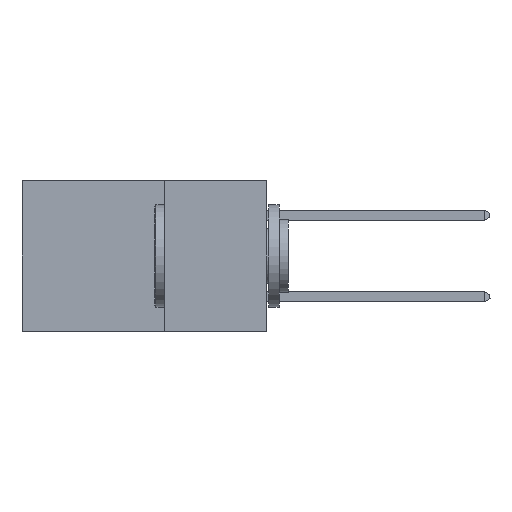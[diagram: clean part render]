
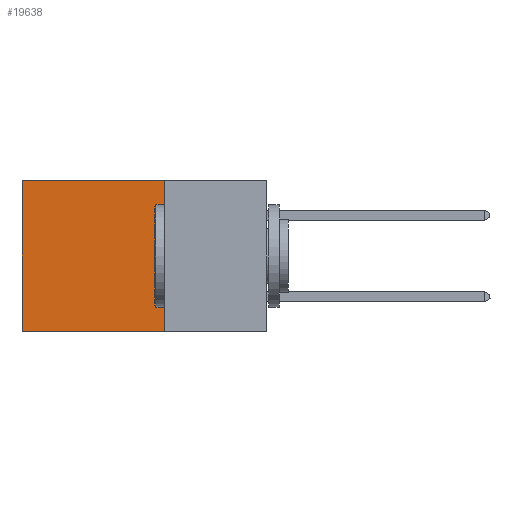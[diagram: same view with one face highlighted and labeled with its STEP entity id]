
A CAD part, left-side view. The second image highlights one B-rep face of the part: STEP entity #19638.
In plain terms, the highlighted planar face has unit normal (-1, 0, 0).
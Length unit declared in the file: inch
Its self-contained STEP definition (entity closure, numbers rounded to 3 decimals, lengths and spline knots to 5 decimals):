
#1198 = ORIENTED_EDGE ( 'NONE', *, *, #2663, .T. ) ;
#2663 = EDGE_CURVE ( 'NONE', #13751, #15221, #23668, .T. ) ;
#2906 = EDGE_CURVE ( 'NONE', #15221, #12397, #26564, .T. ) ;
#3174 = FACE_OUTER_BOUND ( 'NONE', #28540, .T. ) ;
#4516 = VERTEX_POINT ( 'NONE', #23375 ) ;
#7090 = CARTESIAN_POINT ( 'NONE',  ( 0.2875, 0.6, 0. ) ) ;
#7209 = ORIENTED_EDGE ( 'NONE', *, *, #2906, .T. ) ;
#8120 = CARTESIAN_POINT ( 'NONE',  ( 0.2875, 0.6, 0. ) ) ;
#8215 = CARTESIAN_POINT ( 'NONE',  ( 0.2875, 0.6, -0.37 ) ) ;
#9302 = VECTOR ( 'NONE', #12708, 39.37008 ) ;
#10698 = ORIENTED_EDGE ( 'NONE', *, *, #28444, .F. ) ;
#11071 = ORIENTED_EDGE ( 'NONE', *, *, #28566, .F. ) ;
#11108 = LINE ( 'NONE', #13402, #21847 ) ;
#12279 = CARTESIAN_POINT ( 'NONE',  ( 0.2875, 0.25, 0. ) ) ;
#12397 = VERTEX_POINT ( 'NONE', #8215 ) ;
#12650 = DIRECTION ( 'NONE',  ( 0., 0., -1. ) ) ;
#12708 = DIRECTION ( 'NONE',  ( 0., 0., -1. ) ) ;
#13402 = CARTESIAN_POINT ( 'NONE',  ( 0.2875, 0.25, -0.37 ) ) ;
#13601 = LINE ( 'NONE', #21610, #9302 ) ;
#13751 = VERTEX_POINT ( 'NONE', #26639 ) ;
#15221 = VERTEX_POINT ( 'NONE', #7090 ) ;
#15795 = DIRECTION ( 'NONE',  ( 0., 0., -1. ) ) ;
#16866 = DIRECTION ( 'NONE',  ( 0., 1., 0. ) ) ;
#17220 = VECTOR ( 'NONE', #12650, 39.37008 ) ;
#19638 = ADVANCED_FACE ( 'NONE', ( #3174 ), #27024, .F. ) ;
#21610 = CARTESIAN_POINT ( 'NONE',  ( 0.2875, 0.25, 0. ) ) ;
#21847 = VECTOR ( 'NONE', #27473, 39.37008 ) ;
#21892 = VECTOR ( 'NONE', #16866, 39.37008 ) ;
#23375 = CARTESIAN_POINT ( 'NONE',  ( 0.2875, 0.25, -0.37 ) ) ;
#23668 = LINE ( 'NONE', #12279, #21892 ) ;
#23943 = AXIS2_PLACEMENT_3D ( 'NONE', #29539, #26926, #15795 ) ;
#26564 = LINE ( 'NONE', #8120, #17220 ) ;
#26639 = CARTESIAN_POINT ( 'NONE',  ( 0.2875, 0.25, 0. ) ) ;
#26926 = DIRECTION ( 'NONE',  ( 1., 0., 0. ) ) ;
#27024 = PLANE ( 'NONE',  #23943 ) ;
#27473 = DIRECTION ( 'NONE',  ( 0., 1., 0. ) ) ;
#28444 = EDGE_CURVE ( 'NONE', #13751, #4516, #13601, .T. ) ;
#28540 = EDGE_LOOP ( 'NONE', ( #7209, #11071, #10698, #1198 ) ) ;
#28566 = EDGE_CURVE ( 'NONE', #4516, #12397, #11108, .T. ) ;
#29539 = CARTESIAN_POINT ( 'NONE',  ( 0.2875, 0.25, 0. ) ) ;
